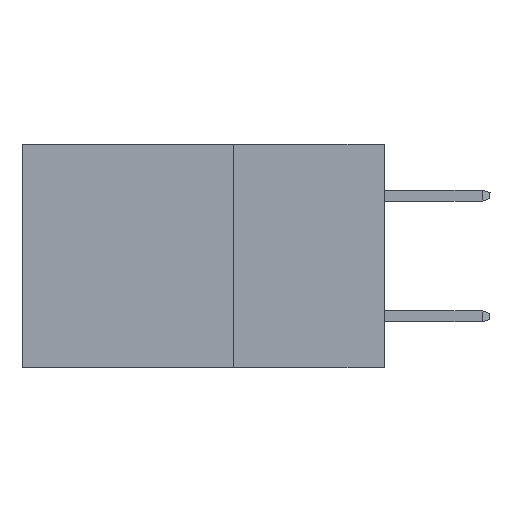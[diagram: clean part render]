
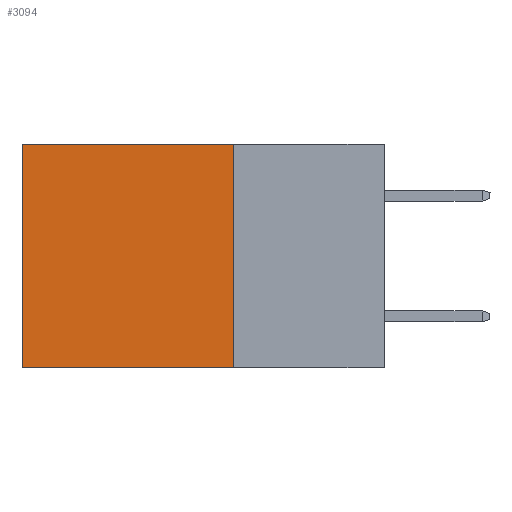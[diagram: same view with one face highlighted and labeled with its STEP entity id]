
A CAD part, left-side view. The second image highlights one B-rep face of the part: STEP entity #3094.
In plain terms, the highlighted planar face has unit normal (-1, 0, 0).
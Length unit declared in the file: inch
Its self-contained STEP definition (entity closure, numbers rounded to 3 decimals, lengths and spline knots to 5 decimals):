
#139 = DIRECTION ( 'NONE',  ( 0., 1., 0. ) ) ;
#640 = LINE ( 'NONE', #20086, #3718 ) ;
#747 = CARTESIAN_POINT ( 'NONE',  ( 0.298, 0.6, 0. ) ) ;
#1262 = LINE ( 'NONE', #10347, #1792 ) ;
#1451 = EDGE_CURVE ( 'NONE', #8415, #13108, #1262, .T. ) ;
#1792 = VECTOR ( 'NONE', #10538, 39.37008 ) ;
#2186 = LINE ( 'NONE', #18937, #12140 ) ;
#2844 = DIRECTION ( 'NONE',  ( 0., 0., -1. ) ) ;
#3094 = ADVANCED_FACE ( 'NONE', ( #7379 ), #13014, .F. ) ;
#3337 = CARTESIAN_POINT ( 'NONE',  ( 0.298, 0.25, -0.37 ) ) ;
#3718 = VECTOR ( 'NONE', #139, 39.37008 ) ;
#4556 = CARTESIAN_POINT ( 'NONE',  ( 0.298, 0.25, 0. ) ) ;
#4937 = CARTESIAN_POINT ( 'NONE',  ( 0.298, 0.6, -0.37 ) ) ;
#7379 = FACE_OUTER_BOUND ( 'NONE', #12027, .T. ) ;
#7659 = DIRECTION ( 'NONE',  ( 1., 0., 0. ) ) ;
#8234 = EDGE_CURVE ( 'NONE', #8415, #14732, #12896, .T. ) ;
#8415 = VERTEX_POINT ( 'NONE', #13179 ) ;
#8953 = DIRECTION ( 'NONE',  ( 0., 0., -1. ) ) ;
#9507 = ORIENTED_EDGE ( 'NONE', *, *, #8234, .T. ) ;
#9630 = ORIENTED_EDGE ( 'NONE', *, *, #16868, .T. ) ;
#10347 = CARTESIAN_POINT ( 'NONE',  ( 0.298, 0.25, 0. ) ) ;
#10538 = DIRECTION ( 'NONE',  ( 0., 0., -1. ) ) ;
#10724 = VERTEX_POINT ( 'NONE', #4937 ) ;
#12027 = EDGE_LOOP ( 'NONE', ( #9630, #18904, #19993, #9507 ) ) ;
#12140 = VECTOR ( 'NONE', #8953, 39.37008 ) ;
#12896 = LINE ( 'NONE', #4556, #14684 ) ;
#13014 = PLANE ( 'NONE',  #16487 ) ;
#13108 = VERTEX_POINT ( 'NONE', #3337 ) ;
#13179 = CARTESIAN_POINT ( 'NONE',  ( 0.298, 0.25, 0. ) ) ;
#14684 = VECTOR ( 'NONE', #21294, 39.37008 ) ;
#14732 = VERTEX_POINT ( 'NONE', #747 ) ;
#16487 = AXIS2_PLACEMENT_3D ( 'NONE', #20635, #7659, #2844 ) ;
#16868 = EDGE_CURVE ( 'NONE', #14732, #10724, #2186, .T. ) ;
#17429 = EDGE_CURVE ( 'NONE', #13108, #10724, #640, .T. ) ;
#18904 = ORIENTED_EDGE ( 'NONE', *, *, #17429, .F. ) ;
#18937 = CARTESIAN_POINT ( 'NONE',  ( 0.298, 0.6, 0. ) ) ;
#19993 = ORIENTED_EDGE ( 'NONE', *, *, #1451, .F. ) ;
#20086 = CARTESIAN_POINT ( 'NONE',  ( 0.298, 0.25, -0.37 ) ) ;
#20635 = CARTESIAN_POINT ( 'NONE',  ( 0.298, 0.25, 0. ) ) ;
#21294 = DIRECTION ( 'NONE',  ( 0., 1., 0. ) ) ;
